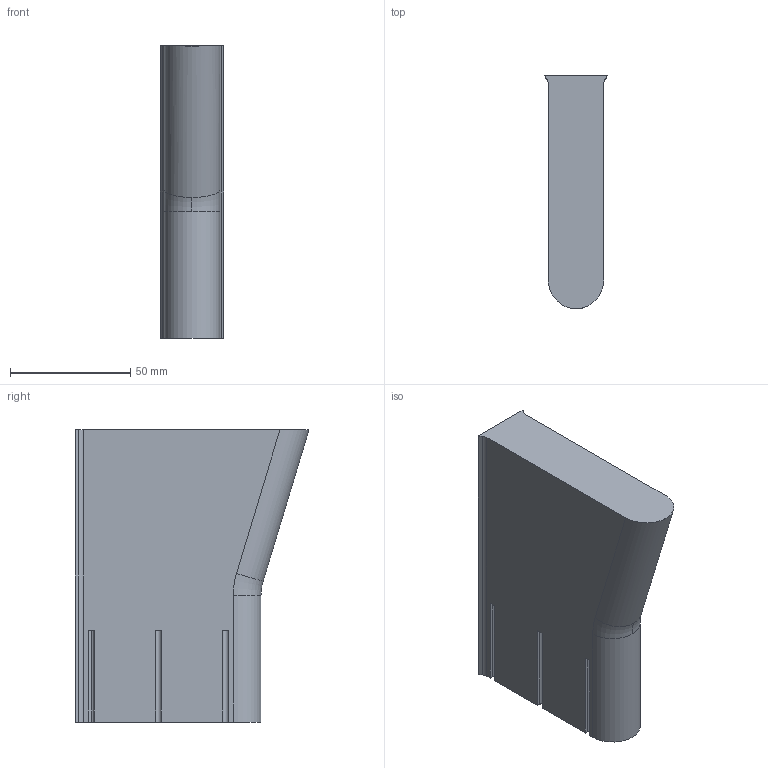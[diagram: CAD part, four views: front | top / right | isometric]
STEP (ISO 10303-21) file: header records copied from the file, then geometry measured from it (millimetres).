
FILE_DESCRIPTION (( 'STEP AP214' ), '1' );
FILE_NAME ('P-15_V2_Part_2.STEP', '2013-12-11T21:50:32', ( 'elpi' ), ( '' ), 'SwSTEP 2.0', 'SolidWorks 2013', '' );
FILE_SCHEMA (( 'AUTOMOTIVE_DESIGN' ));
Length unit declared in the file: inch
Products named in the file (1): P-15_V2_Part_2
Bounding box: 26.28 x 97.04 x 121.3 mm (x, y, z)
Volume: 121363.9 mm3; surface area: 45194.1 mm2
Topology: 1 solids, 1 shells, 47 faces, 135 edges, 88 vertices
Faces by surface type: plane 25, cylinder 17, torus 3, sphere 2
Entity records: 1686 total; most frequent: CARTESIAN_POINT 286, DIRECTION 268, ORIENTED_EDGE 266, EDGE_CURVE 133, AXIS2_PLACEMENT_3D 90, VERTEX_POINT 88, LINE 88, VECTOR 88
